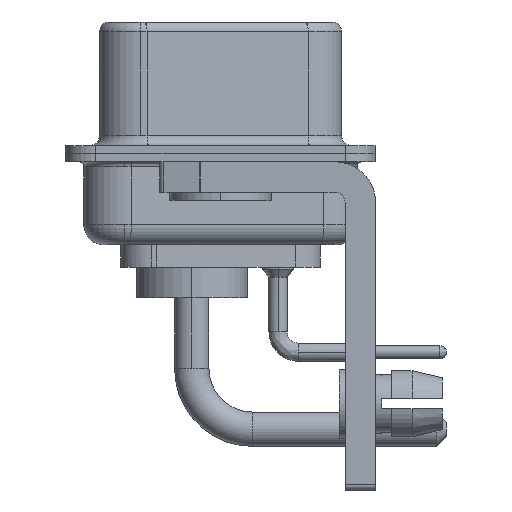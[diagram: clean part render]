
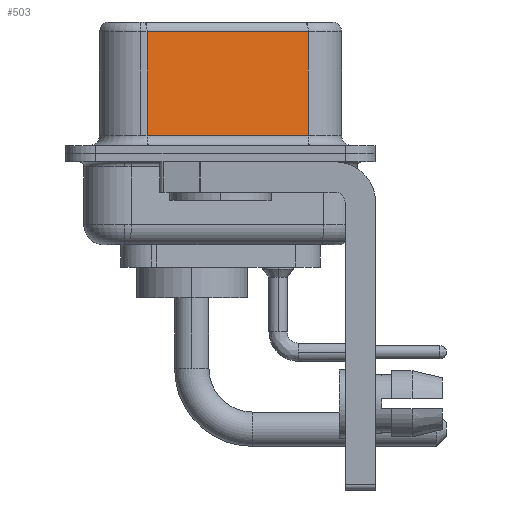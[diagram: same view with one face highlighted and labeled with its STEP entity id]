
A CAD part, left-side view. The second image highlights one B-rep face of the part: STEP entity #503.
In plain terms, the highlighted planar face has unit normal (-0.985, -0.174, 0).
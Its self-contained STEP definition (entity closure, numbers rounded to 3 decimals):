
#503 = ADVANCED_FACE ( 'NONE', ( #13388 ), #3278, .F. ) ;
#991 = VERTEX_POINT ( 'NONE', #11994 ) ;
#1182 = VERTEX_POINT ( 'NONE', #22766 ) ;
#2224 = ORIENTED_EDGE ( 'NONE', *, *, #8432, .T. ) ;
#2640 = DIRECTION ( 'NONE',  ( 0., 0., -1. ) ) ;
#2917 = LINE ( 'NONE', #3048, #22225 ) ;
#3048 = CARTESIAN_POINT ( 'NONE',  ( 5.132, -4.322, 6.52 ) ) ;
#3278 = PLANE ( 'NONE',  #23367 ) ;
#4010 = ORIENTED_EDGE ( 'NONE', *, *, #25628, .T. ) ;
#5609 = VERTEX_POINT ( 'NONE', #15596 ) ;
#6627 = LINE ( 'NONE', #11017, #12317 ) ;
#7405 = DIRECTION ( 'NONE',  ( -0.174, 0.985, 0. ) ) ;
#8231 = VECTOR ( 'NONE', #9106, 1000. ) ;
#8432 = EDGE_CURVE ( 'NONE', #5609, #1182, #6627, .T. ) ;
#9106 = DIRECTION ( 'NONE',  ( 0.174, -0.985, 0. ) ) ;
#9515 = DIRECTION ( 'NONE',  ( -0.174, 0.985, 0. ) ) ;
#11017 = CARTESIAN_POINT ( 'NONE',  ( 3.73, 3.628, 6.52 ) ) ;
#11106 = LINE ( 'NONE', #14715, #8231 ) ;
#11385 = CARTESIAN_POINT ( 'NONE',  ( 5.132, -4.322, 6.52 ) ) ;
#11994 = CARTESIAN_POINT ( 'NONE',  ( 5.132, -4.322, 0.9 ) ) ;
#12317 = VECTOR ( 'NONE', #2640, 1000. ) ;
#12409 = EDGE_CURVE ( 'NONE', #25039, #5609, #25743, .T. ) ;
#13355 = VECTOR ( 'NONE', #7405, 1000. ) ;
#13388 = FACE_OUTER_BOUND ( 'NONE', #16048, .T. ) ;
#13530 = CARTESIAN_POINT ( 'NONE',  ( 5.132, -4.322, 6.02 ) ) ;
#14715 = CARTESIAN_POINT ( 'NONE',  ( 5.132, -4.322, 0.9 ) ) ;
#15596 = CARTESIAN_POINT ( 'NONE',  ( 3.73, 3.628, 6.02 ) ) ;
#16048 = EDGE_LOOP ( 'NONE', ( #20993, #21247, #2224, #4010 ) ) ;
#17444 = DIRECTION ( 'NONE',  ( 0., 0., -1. ) ) ;
#17664 = DIRECTION ( 'NONE',  ( 0.985, 0.174, 0. ) ) ;
#20993 = ORIENTED_EDGE ( 'NONE', *, *, #23397, .F. ) ;
#21247 = ORIENTED_EDGE ( 'NONE', *, *, #12409, .T. ) ;
#22225 = VECTOR ( 'NONE', #17444, 1000. ) ;
#22766 = CARTESIAN_POINT ( 'NONE',  ( 3.73, 3.628, 0.9 ) ) ;
#23367 = AXIS2_PLACEMENT_3D ( 'NONE', #11385, #17664, #9515 ) ;
#23397 = EDGE_CURVE ( 'NONE', #25039, #991, #2917, .T. ) ;
#24715 = CARTESIAN_POINT ( 'NONE',  ( 5.132, -4.322, 6.02 ) ) ;
#25039 = VERTEX_POINT ( 'NONE', #24715 ) ;
#25628 = EDGE_CURVE ( 'NONE', #1182, #991, #11106, .T. ) ;
#25743 = LINE ( 'NONE', #13530, #13355 ) ;
